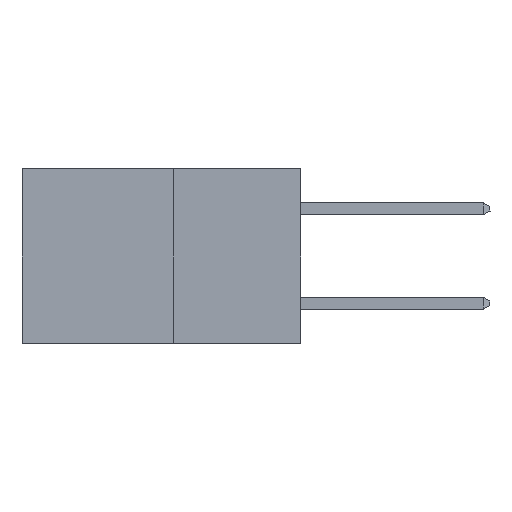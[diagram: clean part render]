
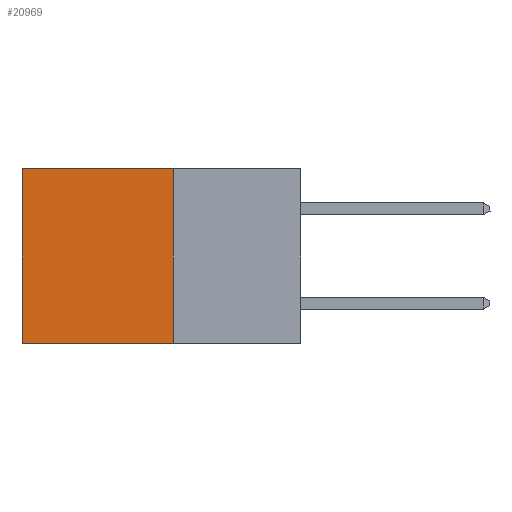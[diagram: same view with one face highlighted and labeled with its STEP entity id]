
A CAD part, left-side view. The second image highlights one B-rep face of the part: STEP entity #20969.
In plain terms, the highlighted planar face has unit normal (-1, 0, 0).
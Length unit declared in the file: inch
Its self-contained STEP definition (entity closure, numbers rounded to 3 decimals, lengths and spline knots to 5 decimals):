
#634 = FACE_OUTER_BOUND ( 'NONE', #15753, .T. ) ;
#1235 = ORIENTED_EDGE ( 'NONE', *, *, #25195, .T. ) ;
#1252 = PLANE ( 'NONE',  #6372 ) ;
#1268 = DIRECTION ( 'NONE',  ( 0., 0., -1. ) ) ;
#2451 = LINE ( 'NONE', #25240, #30184 ) ;
#3907 = DIRECTION ( 'NONE',  ( 0., 0., -1. ) ) ;
#4511 = LINE ( 'NONE', #16923, #17889 ) ;
#5773 = CARTESIAN_POINT ( 'NONE',  ( 0.277, 0.59, -0.37 ) ) ;
#6372 = AXIS2_PLACEMENT_3D ( 'NONE', #28041, #6714, #25439 ) ;
#6400 = LINE ( 'NONE', #31230, #26929 ) ;
#6714 = DIRECTION ( 'NONE',  ( 1., 0., 0. ) ) ;
#7808 = ORIENTED_EDGE ( 'NONE', *, *, #32662, .T. ) ;
#9398 = CARTESIAN_POINT ( 'NONE',  ( 0.277, 0.27, 0. ) ) ;
#9488 = VERTEX_POINT ( 'NONE', #9398 ) ;
#10223 = VECTOR ( 'NONE', #1268, 39.37008 ) ;
#15753 = EDGE_LOOP ( 'NONE', ( #7808, #22139, #32720, #1235 ) ) ;
#16923 = CARTESIAN_POINT ( 'NONE',  ( 0.277, 0.27, -0.37 ) ) ;
#17889 = VECTOR ( 'NONE', #22325, 39.37008 ) ;
#19918 = CARTESIAN_POINT ( 'NONE',  ( 0.277, 0.27, -0.37 ) ) ;
#20178 = EDGE_CURVE ( 'NONE', #22921, #33762, #4511, .T. ) ;
#20969 = ADVANCED_FACE ( 'NONE', ( #634 ), #1252, .F. ) ;
#22139 = ORIENTED_EDGE ( 'NONE', *, *, #20178, .F. ) ;
#22325 = DIRECTION ( 'NONE',  ( 0., 1., 0. ) ) ;
#22921 = VERTEX_POINT ( 'NONE', #28052 ) ;
#23213 = DIRECTION ( 'NONE',  ( 0., 1., 0. ) ) ;
#24476 = LINE ( 'NONE', #19918, #10223 ) ;
#25195 = EDGE_CURVE ( 'NONE', #9488, #31581, #6400, .T. ) ;
#25240 = CARTESIAN_POINT ( 'NONE',  ( 0.277, 0.59, -0.37 ) ) ;
#25439 = DIRECTION ( 'NONE',  ( 0., 0., -1. ) ) ;
#26929 = VECTOR ( 'NONE', #23213, 39.37008 ) ;
#27373 = CARTESIAN_POINT ( 'NONE',  ( 0.277, 0.59, 0. ) ) ;
#28041 = CARTESIAN_POINT ( 'NONE',  ( 0.277, 0.27, -0.37 ) ) ;
#28052 = CARTESIAN_POINT ( 'NONE',  ( 0.277, 0.27, -0.37 ) ) ;
#29773 = EDGE_CURVE ( 'NONE', #9488, #22921, #24476, .T. ) ;
#30184 = VECTOR ( 'NONE', #3907, 39.37008 ) ;
#31230 = CARTESIAN_POINT ( 'NONE',  ( 0.277, 0.27, 0. ) ) ;
#31581 = VERTEX_POINT ( 'NONE', #27373 ) ;
#32662 = EDGE_CURVE ( 'NONE', #31581, #33762, #2451, .T. ) ;
#32720 = ORIENTED_EDGE ( 'NONE', *, *, #29773, .F. ) ;
#33762 = VERTEX_POINT ( 'NONE', #5773 ) ;
